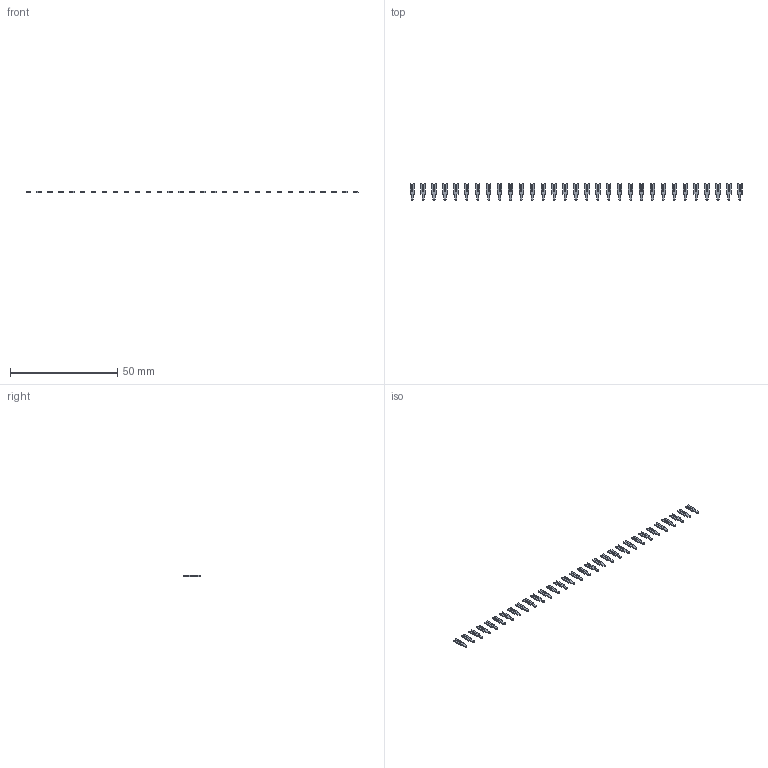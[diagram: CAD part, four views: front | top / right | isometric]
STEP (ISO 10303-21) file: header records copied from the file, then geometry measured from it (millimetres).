
FILE_DESCRIPTION (( 'STEP AP203' ), '1' );
FILE_NAME ('103-031-253-200.STEP', '2020-04-09T20:54:54', ( '' ), ( '' ), 'SwSTEP 2.0', 'SolidWorks 2016', '' );
FILE_SCHEMA (( 'CONFIG_CONTROL_DESIGN' ));
Length unit declared in the file: inch
Products named in the file (2): 103-031-253-200; 100-290-001_100-290-253
Assembly tree (31 placements, depth 2):
  103-031-253-200
    100-290-001_100-290-253  x31
Bounding box: 154.43 x 7.62 x 0.51 mm (x, y, z)
Volume: 171 mm3; surface area: 1066.6 mm2
Topology: 31 solids, 31 shells, 620 faces, 1674 edges, 1116 vertices
Faces by surface type: plane 589, cylinder 31
Entity records: 1780 total; most frequent: DIRECTION 164, CARTESIAN_POINT 144, ORIENTED_EDGE 108, DATE_AND_TIME 72, COORDINATED_UNIVERSAL_TIME_OFFSET 72, CALENDAR_DATE 72, LOCAL_TIME 72, AXIS2_PLACEMENT_3D 56
